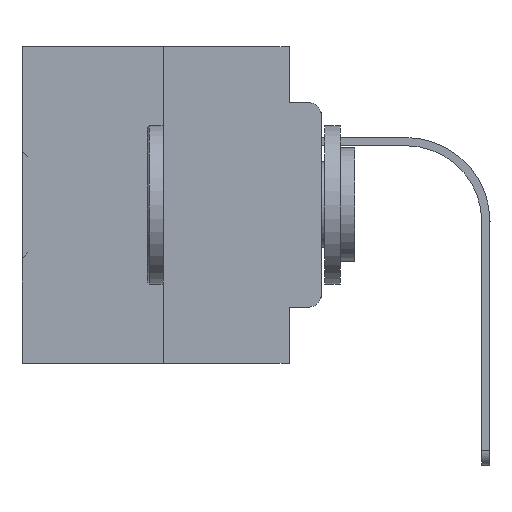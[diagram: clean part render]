
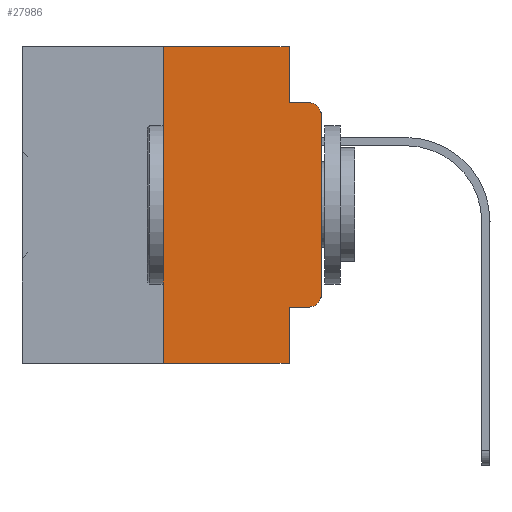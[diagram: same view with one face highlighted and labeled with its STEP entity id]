
A CAD part, left-side view. The second image highlights one B-rep face of the part: STEP entity #27986.
In plain terms, the highlighted planar face has unit normal (-1, 0, 0).
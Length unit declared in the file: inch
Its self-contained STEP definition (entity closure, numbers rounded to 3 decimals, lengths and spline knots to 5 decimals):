
#42 = CARTESIAN_POINT ( 'NONE',  ( 0., 0.051, 0. ) ) ;
#170 = VERTEX_POINT ( 'NONE', #22238 ) ;
#909 = CIRCLE ( 'NONE', #24482, 0.02 ) ;
#1195 = VERTEX_POINT ( 'NONE', #18793 ) ;
#2375 = EDGE_CURVE ( 'NONE', #170, #7883, #31631, .T. ) ;
#2443 = VERTEX_POINT ( 'NONE', #8085 ) ;
#2455 = VECTOR ( 'NONE', #32780, 39.37008 ) ;
#2481 = LINE ( 'NONE', #42, #32963 ) ;
#3462 = DIRECTION ( 'NONE',  ( 0., -1., 0. ) ) ;
#3718 = DIRECTION ( 'NONE',  ( 0., 0., 1. ) ) ;
#4902 = DIRECTION ( 'NONE',  ( 0., 0., -1. ) ) ;
#5045 = EDGE_CURVE ( 'NONE', #16846, #7883, #35791, .T. ) ;
#5659 = EDGE_CURVE ( 'NONE', #31575, #17749, #28343, .T. ) ;
#5847 = DIRECTION ( 'NONE',  ( 0., -1., 0. ) ) ;
#6368 = VERTEX_POINT ( 'NONE', #26510 ) ;
#7189 = CARTESIAN_POINT ( 'NONE',  ( 0., 0.02, -0.1085 ) ) ;
#7883 = VERTEX_POINT ( 'NONE', #17513 ) ;
#8057 = ORIENTED_EDGE ( 'NONE', *, *, #12536, .T. ) ;
#8085 = CARTESIAN_POINT ( 'NONE',  ( 0., 0.051, -0.4115 ) ) ;
#8137 = DIRECTION ( 'NONE',  ( 0., -1., 0. ) ) ;
#9232 = CARTESIAN_POINT ( 'NONE',  ( 0., 0.02, -0.3915 ) ) ;
#10526 = ORIENTED_EDGE ( 'NONE', *, *, #12507, .F. ) ;
#10801 = VECTOR ( 'NONE', #3462, 39.37008 ) ;
#11005 = CARTESIAN_POINT ( 'NONE',  ( 0., 0.25, 0. ) ) ;
#11040 = LINE ( 'NONE', #28358, #25572 ) ;
#11099 = ORIENTED_EDGE ( 'NONE', *, *, #5659, .F. ) ;
#11156 = LINE ( 'NONE', #18781, #2455 ) ;
#11792 = CARTESIAN_POINT ( 'NONE',  ( 0., 0.051, 0. ) ) ;
#12507 = EDGE_CURVE ( 'NONE', #1195, #31575, #28962, .T. ) ;
#12536 = EDGE_CURVE ( 'NONE', #29993, #6368, #909, .T. ) ;
#13403 = EDGE_CURVE ( 'NONE', #6368, #170, #35237, .T. ) ;
#14575 = EDGE_CURVE ( 'NONE', #2443, #30897, #2481, .T. ) ;
#15146 = DIRECTION ( 'NONE',  ( -1., 0., 0. ) ) ;
#15653 = EDGE_CURVE ( 'NONE', #17749, #16846, #25811, .T. ) ;
#15844 = ORIENTED_EDGE ( 'NONE', *, *, #22074, .T. ) ;
#15888 = EDGE_CURVE ( 'NONE', #1195, #30897, #11156, .T. ) ;
#16846 = VERTEX_POINT ( 'NONE', #22682 ) ;
#16963 = ORIENTED_EDGE ( 'NONE', *, *, #14575, .F. ) ;
#17513 = CARTESIAN_POINT ( 'NONE',  ( 0., 0.02, -0.0885 ) ) ;
#17749 = VERTEX_POINT ( 'NONE', #36204 ) ;
#17775 = DIRECTION ( 'NONE',  ( 0., 0., 1. ) ) ;
#18463 = DIRECTION ( 'NONE',  ( -1., 0., 0. ) ) ;
#18781 = CARTESIAN_POINT ( 'NONE',  ( 0., 0.473, -0.5 ) ) ;
#18793 = CARTESIAN_POINT ( 'NONE',  ( 0., 0.25, -0.5 ) ) ;
#22074 = EDGE_CURVE ( 'NONE', #2443, #29993, #11040, .T. ) ;
#22238 = CARTESIAN_POINT ( 'NONE',  ( 0., 0., -0.1085 ) ) ;
#22682 = CARTESIAN_POINT ( 'NONE',  ( 0., 0.051, -0.0885 ) ) ;
#23108 = ORIENTED_EDGE ( 'NONE', *, *, #15653, .F. ) ;
#23122 = VECTOR ( 'NONE', #8137, 39.37008 ) ;
#23795 = CARTESIAN_POINT ( 'NONE',  ( 0., 0.25, 0. ) ) ;
#24154 = EDGE_LOOP ( 'NONE', ( #27315, #30662, #26139, #23108, #11099, #10526, #34663, #16963, #15844, #8057 ) ) ;
#24482 = AXIS2_PLACEMENT_3D ( 'NONE', #9232, #15146, #34459 ) ;
#25051 = DIRECTION ( 'NONE',  ( 1., 0., 0. ) ) ;
#25572 = VECTOR ( 'NONE', #5847, 39.37008 ) ;
#25811 = LINE ( 'NONE', #11792, #35414 ) ;
#26139 = ORIENTED_EDGE ( 'NONE', *, *, #5045, .F. ) ;
#26510 = CARTESIAN_POINT ( 'NONE',  ( 0., 0., -0.3915 ) ) ;
#27275 = CARTESIAN_POINT ( 'NONE',  ( 0., 0.051, -0.5 ) ) ;
#27315 = ORIENTED_EDGE ( 'NONE', *, *, #13403, .T. ) ;
#27986 = ADVANCED_FACE ( 'NONE', ( #30410 ), #30764, .F. ) ;
#28009 = AXIS2_PLACEMENT_3D ( 'NONE', #7189, #18463, #29705 ) ;
#28279 = AXIS2_PLACEMENT_3D ( 'NONE', #35727, #25051, #36076 ) ;
#28343 = LINE ( 'NONE', #28728, #10801 ) ;
#28358 = CARTESIAN_POINT ( 'NONE',  ( 0., 0.051, -0.4115 ) ) ;
#28728 = CARTESIAN_POINT ( 'NONE',  ( 0., 0.473, 0. ) ) ;
#28962 = LINE ( 'NONE', #23795, #32685 ) ;
#29705 = DIRECTION ( 'NONE',  ( 0., 0., -1. ) ) ;
#29993 = VERTEX_POINT ( 'NONE', #32018 ) ;
#30410 = FACE_OUTER_BOUND ( 'NONE', #24154, .T. ) ;
#30662 = ORIENTED_EDGE ( 'NONE', *, *, #2375, .T. ) ;
#30764 = PLANE ( 'NONE',  #28279 ) ;
#30897 = VERTEX_POINT ( 'NONE', #27275 ) ;
#31575 = VERTEX_POINT ( 'NONE', #11005 ) ;
#31631 = CIRCLE ( 'NONE', #28009, 0.02 ) ;
#32018 = CARTESIAN_POINT ( 'NONE',  ( 0., 0.02, -0.4115 ) ) ;
#32685 = VECTOR ( 'NONE', #3718, 39.37008 ) ;
#32780 = DIRECTION ( 'NONE',  ( 0., -1., 0. ) ) ;
#32963 = VECTOR ( 'NONE', #4902, 39.37008 ) ;
#34238 = DIRECTION ( 'NONE',  ( 0., 0., -1. ) ) ;
#34459 = DIRECTION ( 'NONE',  ( 0., 0., -1. ) ) ;
#34663 = ORIENTED_EDGE ( 'NONE', *, *, #15888, .T. ) ;
#34671 = VECTOR ( 'NONE', #17775, 39.37008 ) ;
#35056 = CARTESIAN_POINT ( 'NONE',  ( 0., 0., 0. ) ) ;
#35237 = LINE ( 'NONE', #35056, #34671 ) ;
#35414 = VECTOR ( 'NONE', #34238, 39.37008 ) ;
#35727 = CARTESIAN_POINT ( 'NONE',  ( 0., 0.473, 0. ) ) ;
#35791 = LINE ( 'NONE', #36150, #23122 ) ;
#36076 = DIRECTION ( 'NONE',  ( 0., 0., -1. ) ) ;
#36150 = CARTESIAN_POINT ( 'NONE',  ( 0., 0.051, -0.0885 ) ) ;
#36204 = CARTESIAN_POINT ( 'NONE',  ( 0., 0.051, 0. ) ) ;
